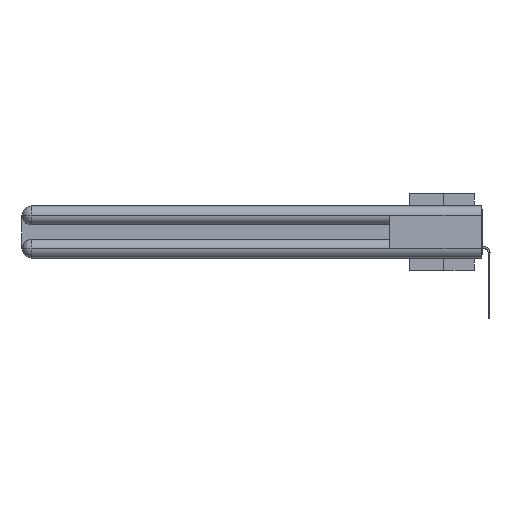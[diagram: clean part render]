
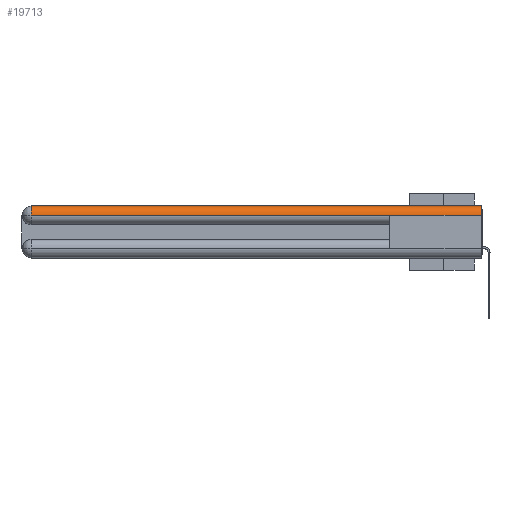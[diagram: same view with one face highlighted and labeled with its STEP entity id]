
A CAD part, left-side view. The second image highlights one B-rep face of the part: STEP entity #19713.
In plain terms, the highlighted cylindrical face has radius 1.562 mm (diameter 3.124 mm), a partial arc.
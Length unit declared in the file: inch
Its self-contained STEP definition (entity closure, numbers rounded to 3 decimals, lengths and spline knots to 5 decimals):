
#366 = CARTESIAN_POINT ( 'NONE',  ( 0., 0.6, -0.0615 ) ) ;
#533 = EDGE_LOOP ( 'NONE', ( #26711, #35285, #24881, #25781, #36746 ) ) ;
#952 = DIRECTION ( 'NONE',  ( 0., 0., 1. ) ) ;
#1105 = CARTESIAN_POINT ( 'NONE',  ( 0.0615, 0., -0.0615 ) ) ;
#2755 = CARTESIAN_POINT ( 'NONE',  ( 0., 2.94, -0.0615 ) ) ;
#3469 = CARTESIAN_POINT ( 'NONE',  ( 0.0615, 0., 0. ) ) ;
#3980 = DIRECTION ( 'NONE',  ( 0., -1., 0. ) ) ;
#4033 = VERTEX_POINT ( 'NONE', #3469 ) ;
#6541 = CARTESIAN_POINT ( 'NONE',  ( 0.0615, 0., -0.0615 ) ) ;
#7675 = LINE ( 'NONE', #29075, #13442 ) ;
#7866 = DIRECTION ( 'NONE',  ( 0., 1., 0. ) ) ;
#8709 = VECTOR ( 'NONE', #31340, 39.37008 ) ;
#12334 = VERTEX_POINT ( 'NONE', #14911 ) ;
#13442 = VECTOR ( 'NONE', #7866, 39.37008 ) ;
#14911 = CARTESIAN_POINT ( 'NONE',  ( 0.0615, 2.94, 0. ) ) ;
#15496 = EDGE_CURVE ( 'NONE', #12334, #28407, #26544, .T. ) ;
#16485 = DIRECTION ( 'NONE',  ( 1., 0., 0. ) ) ;
#19120 = CARTESIAN_POINT ( 'NONE',  ( 0., 3., -0.0615 ) ) ;
#19217 = EDGE_CURVE ( 'NONE', #12334, #4033, #29808, .T. ) ;
#19713 = ADVANCED_FACE ( 'NONE', ( #24731 ), #21524, .T. ) ;
#20633 = CARTESIAN_POINT ( 'NONE',  ( 0., 0., -0.0615 ) ) ;
#21366 = DIRECTION ( 'NONE',  ( 0., -1., 0. ) ) ;
#21524 = CYLINDRICAL_SURFACE ( 'NONE', #32461, 0.0615 ) ;
#22049 = AXIS2_PLACEMENT_3D ( 'NONE', #34779, #3980, #31561 ) ;
#22174 = EDGE_CURVE ( 'NONE', #29294, #24709, #7675, .T. ) ;
#23268 = AXIS2_PLACEMENT_3D ( 'NONE', #1105, #31682, #16485 ) ;
#24709 = VERTEX_POINT ( 'NONE', #366 ) ;
#24731 = FACE_OUTER_BOUND ( 'NONE', #533, .T. ) ;
#24881 = ORIENTED_EDGE ( 'NONE', *, *, #35940, .T. ) ;
#25781 = ORIENTED_EDGE ( 'NONE', *, *, #22174, .F. ) ;
#26544 = CIRCLE ( 'NONE', #22049, 0.0615 ) ;
#26711 = ORIENTED_EDGE ( 'NONE', *, *, #19217, .F. ) ;
#28407 = VERTEX_POINT ( 'NONE', #2755 ) ;
#29075 = CARTESIAN_POINT ( 'NONE',  ( 0., 3., -0.0615 ) ) ;
#29294 = VERTEX_POINT ( 'NONE', #20633 ) ;
#29654 = CIRCLE ( 'NONE', #23268, 0.0615 ) ;
#29808 = LINE ( 'NONE', #33196, #35026 ) ;
#29824 = EDGE_CURVE ( 'NONE', #4033, #29294, #29654, .T. ) ;
#30545 = DIRECTION ( 'NONE',  ( 0., 1., 0. ) ) ;
#31340 = DIRECTION ( 'NONE',  ( 0., -1., 0. ) ) ;
#31561 = DIRECTION ( 'NONE',  ( 0., 0., 1. ) ) ;
#31682 = DIRECTION ( 'NONE',  ( 0., -1., 0. ) ) ;
#32461 = AXIS2_PLACEMENT_3D ( 'NONE', #6541, #30545, #952 ) ;
#33196 = CARTESIAN_POINT ( 'NONE',  ( 0.0615, 0., 0. ) ) ;
#34779 = CARTESIAN_POINT ( 'NONE',  ( 0.0615, 2.94, -0.0615 ) ) ;
#35026 = VECTOR ( 'NONE', #21366, 39.37008 ) ;
#35285 = ORIENTED_EDGE ( 'NONE', *, *, #15496, .T. ) ;
#35940 = EDGE_CURVE ( 'NONE', #28407, #24709, #36743, .T. ) ;
#36743 = LINE ( 'NONE', #19120, #8709 ) ;
#36746 = ORIENTED_EDGE ( 'NONE', *, *, #29824, .F. ) ;
